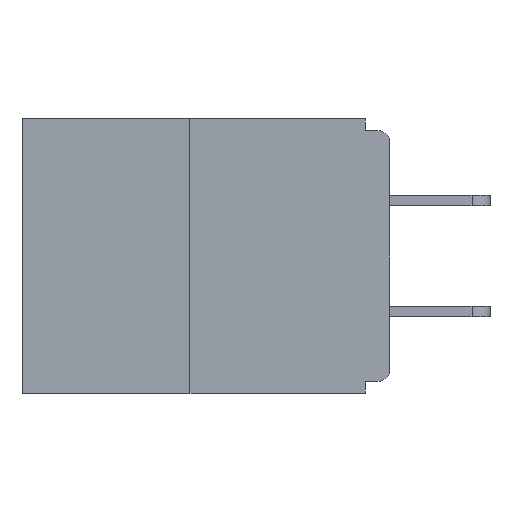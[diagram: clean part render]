
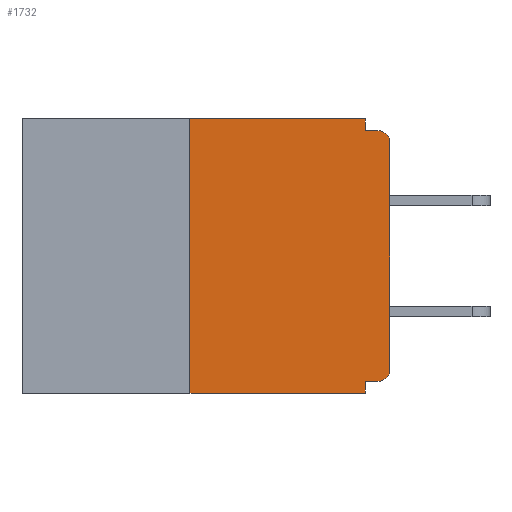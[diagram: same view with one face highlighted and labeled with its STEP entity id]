
A CAD part, left-side view. The second image highlights one B-rep face of the part: STEP entity #1732.
In plain terms, the highlighted planar face has unit normal (-1, 0, 0).
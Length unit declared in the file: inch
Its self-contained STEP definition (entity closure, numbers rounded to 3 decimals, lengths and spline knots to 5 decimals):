
#144 = VECTOR ( 'NONE', #6872, 39.37008 ) ;
#229 = FACE_OUTER_BOUND ( 'NONE', #4336, .T. ) ;
#285 = ORIENTED_EDGE ( 'NONE', *, *, #2772, .F. ) ;
#416 = VECTOR ( 'NONE', #6843, 39.37008 ) ;
#762 = CARTESIAN_POINT ( 'NONE',  ( 0., 0.015, -0.015 ) ) ;
#1080 = CARTESIAN_POINT ( 'NONE',  ( 0., 0.031, -0.343 ) ) ;
#1346 = LINE ( 'NONE', #14150, #9658 ) ;
#1474 = ORIENTED_EDGE ( 'NONE', *, *, #1938, .T. ) ;
#1683 = CARTESIAN_POINT ( 'NONE',  ( 0., 0.031, 0. ) ) ;
#1732 = ADVANCED_FACE ( 'NONE', ( #229 ), #9713, .F. ) ;
#1938 = EDGE_CURVE ( 'NONE', #11835, #7740, #13275, .T. ) ;
#2591 = DIRECTION ( 'NONE',  ( 0., 0., 1. ) ) ;
#2739 = EDGE_CURVE ( 'NONE', #14096, #13559, #6190, .T. ) ;
#2772 = EDGE_CURVE ( 'NONE', #4124, #4006, #9177, .T. ) ;
#2806 = DIRECTION ( 'NONE',  ( 0., 0., -1. ) ) ;
#3235 = CARTESIAN_POINT ( 'NONE',  ( 0., 0.46, -0.343 ) ) ;
#3690 = VERTEX_POINT ( 'NONE', #12710 ) ;
#4006 = VERTEX_POINT ( 'NONE', #13449 ) ;
#4124 = VERTEX_POINT ( 'NONE', #11370 ) ;
#4160 = EDGE_CURVE ( 'NONE', #4006, #14096, #5420, .T. ) ;
#4271 = DIRECTION ( 'NONE',  ( 0., -1., 0. ) ) ;
#4283 = ORIENTED_EDGE ( 'NONE', *, *, #12558, .T. ) ;
#4336 = EDGE_LOOP ( 'NONE', ( #4652, #285, #4283, #12186, #8236, #11148, #1474, #12129, #4370, #14586 ) ) ;
#4370 = ORIENTED_EDGE ( 'NONE', *, *, #12377, .F. ) ;
#4454 = AXIS2_PLACEMENT_3D ( 'NONE', #10754, #14306, #14453 ) ;
#4652 = ORIENTED_EDGE ( 'NONE', *, *, #4160, .F. ) ;
#4872 = EDGE_CURVE ( 'NONE', #3690, #12694, #1346, .T. ) ;
#4921 = DIRECTION ( 'NONE',  ( -1., 0., 0. ) ) ;
#4964 = VECTOR ( 'NONE', #6693, 39.37008 ) ;
#5064 = CIRCLE ( 'NONE', #4454, 0.015 ) ;
#5401 = DIRECTION ( 'NONE',  ( 0., -1., 0. ) ) ;
#5420 = LINE ( 'NONE', #12518, #144 ) ;
#5933 = LINE ( 'NONE', #8742, #8046 ) ;
#6190 = LINE ( 'NONE', #1683, #6887 ) ;
#6557 = CARTESIAN_POINT ( 'NONE',  ( 0., 0., -0.313 ) ) ;
#6627 = AXIS2_PLACEMENT_3D ( 'NONE', #14026, #4921, #12796 ) ;
#6693 = DIRECTION ( 'NONE',  ( 0., 0., 1. ) ) ;
#6698 = EDGE_CURVE ( 'NONE', #3690, #11835, #5064, .T. ) ;
#6766 = CARTESIAN_POINT ( 'NONE',  ( 0., 0.031, -0.015 ) ) ;
#6833 = CARTESIAN_POINT ( 'NONE',  ( 0., 0., 0. ) ) ;
#6843 = DIRECTION ( 'NONE',  ( 0., 0., -1. ) ) ;
#6872 = DIRECTION ( 'NONE',  ( 0., -1., 0. ) ) ;
#6887 = VECTOR ( 'NONE', #6962, 39.37008 ) ;
#6962 = DIRECTION ( 'NONE',  ( 0., 0., -1. ) ) ;
#7291 = DIRECTION ( 'NONE',  ( 1., 0., 0. ) ) ;
#7740 = VERTEX_POINT ( 'NONE', #12113 ) ;
#8046 = VECTOR ( 'NONE', #4271, 39.37008 ) ;
#8236 = ORIENTED_EDGE ( 'NONE', *, *, #4872, .F. ) ;
#8271 = CIRCLE ( 'NONE', #6627, 0.015 ) ;
#8631 = VERTEX_POINT ( 'NONE', #762 ) ;
#8742 = CARTESIAN_POINT ( 'NONE',  ( 0., 0., -0.015 ) ) ;
#9177 = LINE ( 'NONE', #13774, #11827 ) ;
#9488 = EDGE_CURVE ( 'NONE', #12694, #14384, #12242, .T. ) ;
#9658 = VECTOR ( 'NONE', #12723, 39.37008 ) ;
#9713 = PLANE ( 'NONE',  #12750 ) ;
#10754 = CARTESIAN_POINT ( 'NONE',  ( 0., 0.015, -0.313 ) ) ;
#11148 = ORIENTED_EDGE ( 'NONE', *, *, #6698, .T. ) ;
#11370 = CARTESIAN_POINT ( 'NONE',  ( 0., 0.25, -0.343 ) ) ;
#11553 = EDGE_CURVE ( 'NONE', #7740, #8631, #8271, .T. ) ;
#11555 = VECTOR ( 'NONE', #5401, 39.37008 ) ;
#11584 = CARTESIAN_POINT ( 'NONE',  ( 0., 0.031, -0.343 ) ) ;
#11827 = VECTOR ( 'NONE', #2591, 39.37008 ) ;
#11835 = VERTEX_POINT ( 'NONE', #6557 ) ;
#12113 = CARTESIAN_POINT ( 'NONE',  ( 0., 0., -0.03 ) ) ;
#12129 = ORIENTED_EDGE ( 'NONE', *, *, #11553, .T. ) ;
#12186 = ORIENTED_EDGE ( 'NONE', *, *, #9488, .F. ) ;
#12242 = LINE ( 'NONE', #1080, #416 ) ;
#12277 = LINE ( 'NONE', #3235, #11555 ) ;
#12377 = EDGE_CURVE ( 'NONE', #13559, #8631, #5933, .T. ) ;
#12420 = CARTESIAN_POINT ( 'NONE',  ( 0., 0.031, -0.328 ) ) ;
#12518 = CARTESIAN_POINT ( 'NONE',  ( 0., 0.46, 0. ) ) ;
#12558 = EDGE_CURVE ( 'NONE', #4124, #14384, #12277, .T. ) ;
#12694 = VERTEX_POINT ( 'NONE', #12420 ) ;
#12710 = CARTESIAN_POINT ( 'NONE',  ( 0., 0.015, -0.328 ) ) ;
#12723 = DIRECTION ( 'NONE',  ( 0., 1., 0. ) ) ;
#12750 = AXIS2_PLACEMENT_3D ( 'NONE', #14235, #7291, #2806 ) ;
#12796 = DIRECTION ( 'NONE',  ( 0., 0., -1. ) ) ;
#13275 = LINE ( 'NONE', #6833, #4964 ) ;
#13449 = CARTESIAN_POINT ( 'NONE',  ( 0., 0.25, 0. ) ) ;
#13559 = VERTEX_POINT ( 'NONE', #6766 ) ;
#13774 = CARTESIAN_POINT ( 'NONE',  ( 0., 0.25, 0. ) ) ;
#14026 = CARTESIAN_POINT ( 'NONE',  ( 0., 0.015, -0.03 ) ) ;
#14096 = VERTEX_POINT ( 'NONE', #14349 ) ;
#14150 = CARTESIAN_POINT ( 'NONE',  ( 0., 0., -0.328 ) ) ;
#14235 = CARTESIAN_POINT ( 'NONE',  ( 0., 0.46, 0. ) ) ;
#14306 = DIRECTION ( 'NONE',  ( -1., 0., 0. ) ) ;
#14349 = CARTESIAN_POINT ( 'NONE',  ( 0., 0.031, 0. ) ) ;
#14384 = VERTEX_POINT ( 'NONE', #11584 ) ;
#14453 = DIRECTION ( 'NONE',  ( 0., 0., -1. ) ) ;
#14586 = ORIENTED_EDGE ( 'NONE', *, *, #2739, .F. ) ;
